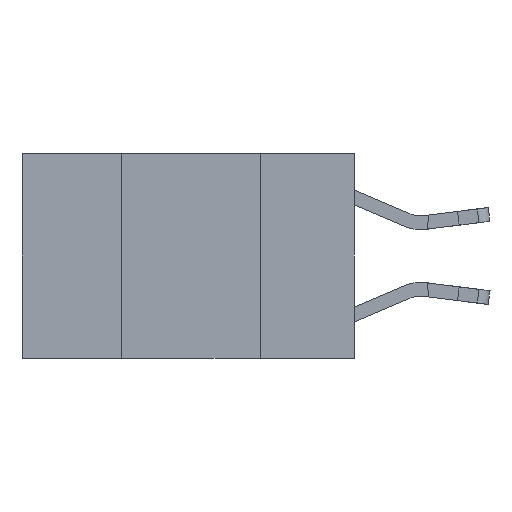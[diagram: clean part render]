
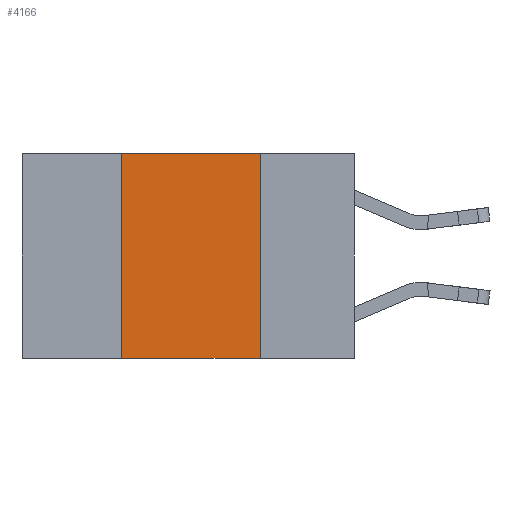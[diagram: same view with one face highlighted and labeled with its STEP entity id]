
A CAD part, left-side view. The second image highlights one B-rep face of the part: STEP entity #4166.
In plain terms, the highlighted planar face has unit normal (-1, 0, 0).
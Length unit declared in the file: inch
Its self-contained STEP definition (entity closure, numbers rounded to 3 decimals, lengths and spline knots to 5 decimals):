
#88 = CARTESIAN_POINT ( 'NONE',  ( 0., 0.6, -0.37 ) ) ;
#120 = VERTEX_POINT ( 'NONE', #7455 ) ;
#200 = CARTESIAN_POINT ( 'NONE',  ( 0., 0.17, 0. ) ) ;
#224 = VECTOR ( 'NONE', #8319, 39.37008 ) ;
#359 = EDGE_CURVE ( 'NONE', #1856, #3483, #11258, .T. ) ;
#804 = AXIS2_PLACEMENT_3D ( 'NONE', #9836, #10840, #4706 ) ;
#1169 = ORIENTED_EDGE ( 'NONE', *, *, #8507, .T. ) ;
#1257 = FACE_OUTER_BOUND ( 'NONE', #7330, .T. ) ;
#1856 = VERTEX_POINT ( 'NONE', #9584 ) ;
#2496 = ORIENTED_EDGE ( 'NONE', *, *, #8752, .F. ) ;
#2649 = PLANE ( 'NONE',  #804 ) ;
#3116 = LINE ( 'NONE', #7678, #5506 ) ;
#3483 = VERTEX_POINT ( 'NONE', #10995 ) ;
#4166 = ADVANCED_FACE ( 'NONE', ( #1257 ), #2649, .F. ) ;
#4706 = DIRECTION ( 'NONE',  ( 0., 0., -1. ) ) ;
#5018 = ORIENTED_EDGE ( 'NONE', *, *, #10166, .F. ) ;
#5506 = VECTOR ( 'NONE', #6678, 39.37008 ) ;
#6351 = DIRECTION ( 'NONE',  ( 0., 0., -1. ) ) ;
#6678 = DIRECTION ( 'NONE',  ( 0., 0., 1. ) ) ;
#7330 = EDGE_LOOP ( 'NONE', ( #5018, #10837, #2496, #1169 ) ) ;
#7455 = CARTESIAN_POINT ( 'NONE',  ( 0., 0.42, -0.37 ) ) ;
#7578 = LINE ( 'NONE', #200, #12957 ) ;
#7678 = CARTESIAN_POINT ( 'NONE',  ( 0., 0.42, 0. ) ) ;
#7923 = VECTOR ( 'NONE', #11265, 39.37008 ) ;
#8319 = DIRECTION ( 'NONE',  ( 0., -1., 0. ) ) ;
#8507 = EDGE_CURVE ( 'NONE', #120, #13000, #11119, .T. ) ;
#8752 = EDGE_CURVE ( 'NONE', #120, #1856, #3116, .T. ) ;
#9584 = CARTESIAN_POINT ( 'NONE',  ( 0., 0.42, 0. ) ) ;
#9836 = CARTESIAN_POINT ( 'NONE',  ( 0., 0.6, 0. ) ) ;
#10166 = EDGE_CURVE ( 'NONE', #3483, #13000, #7578, .T. ) ;
#10837 = ORIENTED_EDGE ( 'NONE', *, *, #359, .F. ) ;
#10840 = DIRECTION ( 'NONE',  ( 1., 0., 0. ) ) ;
#10995 = CARTESIAN_POINT ( 'NONE',  ( 0., 0.17, 0. ) ) ;
#11058 = CARTESIAN_POINT ( 'NONE',  ( 0., 0.17, -0.37 ) ) ;
#11119 = LINE ( 'NONE', #88, #224 ) ;
#11258 = LINE ( 'NONE', #11652, #7923 ) ;
#11265 = DIRECTION ( 'NONE',  ( 0., -1., 0. ) ) ;
#11652 = CARTESIAN_POINT ( 'NONE',  ( 0., 0.6, 0. ) ) ;
#12957 = VECTOR ( 'NONE', #6351, 39.37008 ) ;
#13000 = VERTEX_POINT ( 'NONE', #11058 ) ;
